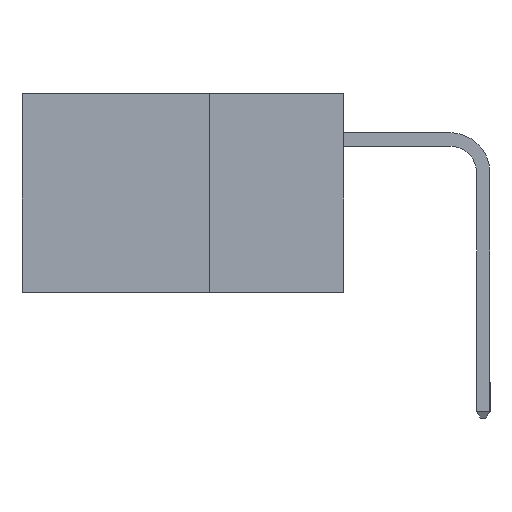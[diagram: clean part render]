
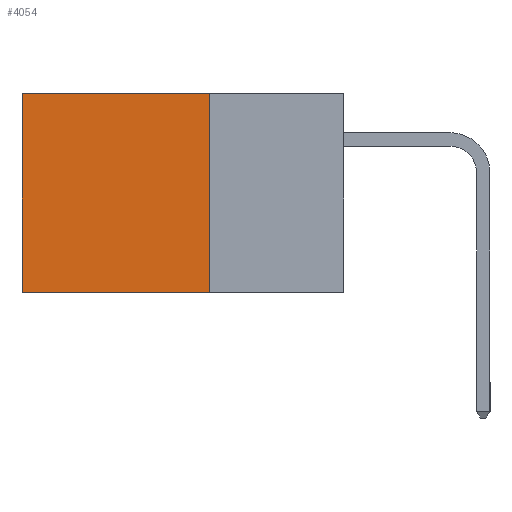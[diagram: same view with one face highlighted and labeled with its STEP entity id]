
A CAD part, left-side view. The second image highlights one B-rep face of the part: STEP entity #4054.
In plain terms, the highlighted planar face has unit normal (-1, 0, 0).
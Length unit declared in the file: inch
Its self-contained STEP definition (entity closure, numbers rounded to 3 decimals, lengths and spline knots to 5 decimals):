
#412 = VECTOR ( 'NONE', #11543, 39.37008 ) ;
#474 = LINE ( 'NONE', #9930, #9952 ) ;
#848 = VECTOR ( 'NONE', #8358, 39.37008 ) ;
#854 = EDGE_CURVE ( 'NONE', #6833, #2004, #10555, .T. ) ;
#909 = DIRECTION ( 'NONE',  ( 0., 0., -1. ) ) ;
#992 = EDGE_CURVE ( 'NONE', #5677, #10329, #474, .T. ) ;
#1398 = DIRECTION ( 'NONE',  ( 0., 0., -1. ) ) ;
#2004 = VERTEX_POINT ( 'NONE', #8286 ) ;
#2475 = VECTOR ( 'NONE', #6221, 39.37008 ) ;
#3500 = CARTESIAN_POINT ( 'NONE',  ( 0.2615, 0.25, -0.37 ) ) ;
#4054 = ADVANCED_FACE ( 'NONE', ( #4516 ), #9435, .F. ) ;
#4516 = FACE_OUTER_BOUND ( 'NONE', #8112, .T. ) ;
#5677 = VERTEX_POINT ( 'NONE', #7360 ) ;
#6221 = DIRECTION ( 'NONE',  ( 0., 1., 0. ) ) ;
#6547 = LINE ( 'NONE', #3500, #848 ) ;
#6833 = VERTEX_POINT ( 'NONE', #7940 ) ;
#7360 = CARTESIAN_POINT ( 'NONE',  ( 0.2615, 0.6, 0. ) ) ;
#7635 = ORIENTED_EDGE ( 'NONE', *, *, #854, .F. ) ;
#7741 = CARTESIAN_POINT ( 'NONE',  ( 0.2615, 0.25, -0.37 ) ) ;
#7940 = CARTESIAN_POINT ( 'NONE',  ( 0.2615, 0.25, 0. ) ) ;
#8112 = EDGE_LOOP ( 'NONE', ( #8512, #9306, #7635, #11481 ) ) ;
#8286 = CARTESIAN_POINT ( 'NONE',  ( 0.2615, 0.25, -0.37 ) ) ;
#8287 = CARTESIAN_POINT ( 'NONE',  ( 0.2615, 0.6, -0.37 ) ) ;
#8313 = CARTESIAN_POINT ( 'NONE',  ( 0.2615, 0.25, -0.37 ) ) ;
#8358 = DIRECTION ( 'NONE',  ( 0., 1., 0. ) ) ;
#8512 = ORIENTED_EDGE ( 'NONE', *, *, #992, .T. ) ;
#9029 = CARTESIAN_POINT ( 'NONE',  ( 0.2615, 0.25, 0. ) ) ;
#9306 = ORIENTED_EDGE ( 'NONE', *, *, #9920, .F. ) ;
#9435 = PLANE ( 'NONE',  #10227 ) ;
#9920 = EDGE_CURVE ( 'NONE', #2004, #10329, #6547, .T. ) ;
#9930 = CARTESIAN_POINT ( 'NONE',  ( 0.2615, 0.6, -0.37 ) ) ;
#9952 = VECTOR ( 'NONE', #1398, 39.37008 ) ;
#10227 = AXIS2_PLACEMENT_3D ( 'NONE', #8313, #12093, #909 ) ;
#10329 = VERTEX_POINT ( 'NONE', #8287 ) ;
#10555 = LINE ( 'NONE', #7741, #412 ) ;
#11013 = LINE ( 'NONE', #9029, #2475 ) ;
#11481 = ORIENTED_EDGE ( 'NONE', *, *, #12085, .T. ) ;
#11543 = DIRECTION ( 'NONE',  ( 0., 0., -1. ) ) ;
#12085 = EDGE_CURVE ( 'NONE', #6833, #5677, #11013, .T. ) ;
#12093 = DIRECTION ( 'NONE',  ( 1., 0., 0. ) ) ;
